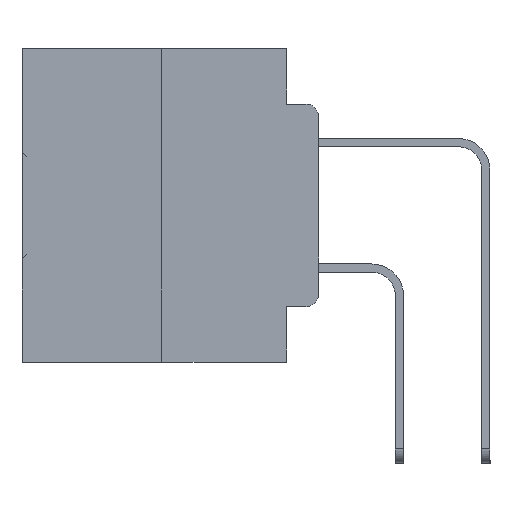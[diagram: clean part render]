
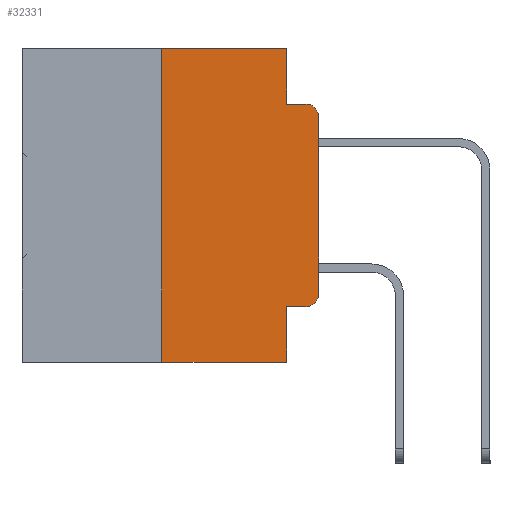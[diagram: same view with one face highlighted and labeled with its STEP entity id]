
A CAD part, left-side view. The second image highlights one B-rep face of the part: STEP entity #32331.
In plain terms, the highlighted planar face has unit normal (-1, 0, 0).
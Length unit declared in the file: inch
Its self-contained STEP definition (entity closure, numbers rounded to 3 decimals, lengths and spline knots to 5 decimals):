
#1193 = AXIS2_PLACEMENT_3D ( 'NONE', #29631, #13144, #32408 ) ;
#1638 = ORIENTED_EDGE ( 'NONE', *, *, #28938, .F. ) ;
#2658 = DIRECTION ( 'NONE',  ( -1., 0., 0. ) ) ;
#3309 = DIRECTION ( 'NONE',  ( 0., -1., 0. ) ) ;
#3437 = VERTEX_POINT ( 'NONE', #4916 ) ;
#3550 = DIRECTION ( 'NONE',  ( 0., -1., 0. ) ) ;
#3716 = LINE ( 'NONE', #34785, #10438 ) ;
#4916 = CARTESIAN_POINT ( 'NONE',  ( 0., 0.051, -0.0885 ) ) ;
#4925 = CARTESIAN_POINT ( 'NONE',  ( 0., 0.473, 0. ) ) ;
#5348 = CIRCLE ( 'NONE', #1193, 0.02 ) ;
#7107 = ORIENTED_EDGE ( 'NONE', *, *, #20678, .T. ) ;
#7170 = EDGE_LOOP ( 'NONE', ( #14008, #15725, #1638, #32140, #17466, #11893, #33855, #12759, #24875, #7107 ) ) ;
#7205 = VERTEX_POINT ( 'NONE', #28105 ) ;
#7998 = CARTESIAN_POINT ( 'NONE',  ( 0., 0.051, 0. ) ) ;
#8064 = LINE ( 'NONE', #34013, #28301 ) ;
#8222 = CARTESIAN_POINT ( 'NONE',  ( 0., 0.25, -0.5 ) ) ;
#9102 = CARTESIAN_POINT ( 'NONE',  ( 0., 0.051, -0.4115 ) ) ;
#9454 = EDGE_CURVE ( 'NONE', #26717, #31744, #16726, .T. ) ;
#10438 = VECTOR ( 'NONE', #18297, 39.37008 ) ;
#10468 = DIRECTION ( 'NONE',  ( 1., 0., 0. ) ) ;
#11393 = CARTESIAN_POINT ( 'NONE',  ( 0., 0.02, -0.4115 ) ) ;
#11823 = EDGE_CURVE ( 'NONE', #12777, #26717, #17229, .T. ) ;
#11893 = ORIENTED_EDGE ( 'NONE', *, *, #20057, .F. ) ;
#12759 = ORIENTED_EDGE ( 'NONE', *, *, #17558, .F. ) ;
#12777 = VERTEX_POINT ( 'NONE', #26662 ) ;
#13144 = DIRECTION ( 'NONE',  ( -1., 0., 0. ) ) ;
#13699 = VECTOR ( 'NONE', #19203, 39.37008 ) ;
#13711 = DIRECTION ( 'NONE',  ( 0., 0., 1. ) ) ;
#14008 = ORIENTED_EDGE ( 'NONE', *, *, #11823, .T. ) ;
#14186 = VECTOR ( 'NONE', #21720, 39.37008 ) ;
#14216 = FACE_OUTER_BOUND ( 'NONE', #7170, .T. ) ;
#14297 = VERTEX_POINT ( 'NONE', #7998 ) ;
#14541 = LINE ( 'NONE', #30044, #13699 ) ;
#15042 = LINE ( 'NONE', #4925, #14186 ) ;
#15725 = ORIENTED_EDGE ( 'NONE', *, *, #9454, .T. ) ;
#16488 = AXIS2_PLACEMENT_3D ( 'NONE', #19439, #2658, #22218 ) ;
#16726 = CIRCLE ( 'NONE', #16488, 0.02 ) ;
#17229 = LINE ( 'NONE', #32982, #30189 ) ;
#17466 = ORIENTED_EDGE ( 'NONE', *, *, #27374, .F. ) ;
#17558 = EDGE_CURVE ( 'NONE', #34787, #19569, #21245, .T. ) ;
#18297 = DIRECTION ( 'NONE',  ( 0., 0., -1. ) ) ;
#18584 = CARTESIAN_POINT ( 'NONE',  ( 0., 0.25, 0. ) ) ;
#18618 = CARTESIAN_POINT ( 'NONE',  ( 0., 0.473, 0. ) ) ;
#19203 = DIRECTION ( 'NONE',  ( 0., -1., 0. ) ) ;
#19439 = CARTESIAN_POINT ( 'NONE',  ( 0., 0.02, -0.1085 ) ) ;
#19569 = VERTEX_POINT ( 'NONE', #24798 ) ;
#19759 = LINE ( 'NONE', #18584, #33526 ) ;
#20057 = EDGE_CURVE ( 'NONE', #31256, #7205, #19759, .T. ) ;
#20212 = EDGE_CURVE ( 'NONE', #31256, #19569, #14541, .T. ) ;
#20678 = EDGE_CURVE ( 'NONE', #22198, #12777, #5348, .T. ) ;
#21245 = LINE ( 'NONE', #29586, #35008 ) ;
#21375 = DIRECTION ( 'NONE',  ( 0., 0., 1. ) ) ;
#21720 = DIRECTION ( 'NONE',  ( 0., -1., 0. ) ) ;
#22084 = CARTESIAN_POINT ( 'NONE',  ( 0., 0.051, -0.4115 ) ) ;
#22198 = VERTEX_POINT ( 'NONE', #11393 ) ;
#22218 = DIRECTION ( 'NONE',  ( 0., 0., -1. ) ) ;
#23269 = VECTOR ( 'NONE', #3309, 39.37008 ) ;
#23924 = CARTESIAN_POINT ( 'NONE',  ( 0., 0., -0.1085 ) ) ;
#24141 = LINE ( 'NONE', #9102, #23269 ) ;
#24798 = CARTESIAN_POINT ( 'NONE',  ( 0., 0.051, -0.5 ) ) ;
#24875 = ORIENTED_EDGE ( 'NONE', *, *, #32688, .T. ) ;
#25111 = AXIS2_PLACEMENT_3D ( 'NONE', #18618, #10468, #29699 ) ;
#26662 = CARTESIAN_POINT ( 'NONE',  ( 0., 0., -0.3915 ) ) ;
#26717 = VERTEX_POINT ( 'NONE', #23924 ) ;
#26814 = DIRECTION ( 'NONE',  ( 0., 0., -1. ) ) ;
#27374 = EDGE_CURVE ( 'NONE', #7205, #14297, #15042, .T. ) ;
#28105 = CARTESIAN_POINT ( 'NONE',  ( 0., 0.25, 0. ) ) ;
#28301 = VECTOR ( 'NONE', #3550, 39.37008 ) ;
#28938 = EDGE_CURVE ( 'NONE', #3437, #31744, #8064, .T. ) ;
#29139 = CARTESIAN_POINT ( 'NONE',  ( 0., 0.02, -0.0885 ) ) ;
#29577 = PLANE ( 'NONE',  #25111 ) ;
#29586 = CARTESIAN_POINT ( 'NONE',  ( 0., 0.051, 0. ) ) ;
#29631 = CARTESIAN_POINT ( 'NONE',  ( 0., 0.02, -0.3915 ) ) ;
#29699 = DIRECTION ( 'NONE',  ( 0., 0., -1. ) ) ;
#30044 = CARTESIAN_POINT ( 'NONE',  ( 0., 0.473, -0.5 ) ) ;
#30189 = VECTOR ( 'NONE', #13711, 39.37008 ) ;
#31256 = VERTEX_POINT ( 'NONE', #8222 ) ;
#31743 = EDGE_CURVE ( 'NONE', #14297, #3437, #3716, .T. ) ;
#31744 = VERTEX_POINT ( 'NONE', #29139 ) ;
#32140 = ORIENTED_EDGE ( 'NONE', *, *, #31743, .F. ) ;
#32331 = ADVANCED_FACE ( 'NONE', ( #14216 ), #29577, .F. ) ;
#32408 = DIRECTION ( 'NONE',  ( 0., 0., -1. ) ) ;
#32688 = EDGE_CURVE ( 'NONE', #34787, #22198, #24141, .T. ) ;
#32982 = CARTESIAN_POINT ( 'NONE',  ( 0., 0., 0. ) ) ;
#33526 = VECTOR ( 'NONE', #21375, 39.37008 ) ;
#33855 = ORIENTED_EDGE ( 'NONE', *, *, #20212, .T. ) ;
#34013 = CARTESIAN_POINT ( 'NONE',  ( 0., 0.051, -0.0885 ) ) ;
#34785 = CARTESIAN_POINT ( 'NONE',  ( 0., 0.051, 0. ) ) ;
#34787 = VERTEX_POINT ( 'NONE', #22084 ) ;
#35008 = VECTOR ( 'NONE', #26814, 39.37008 ) ;
